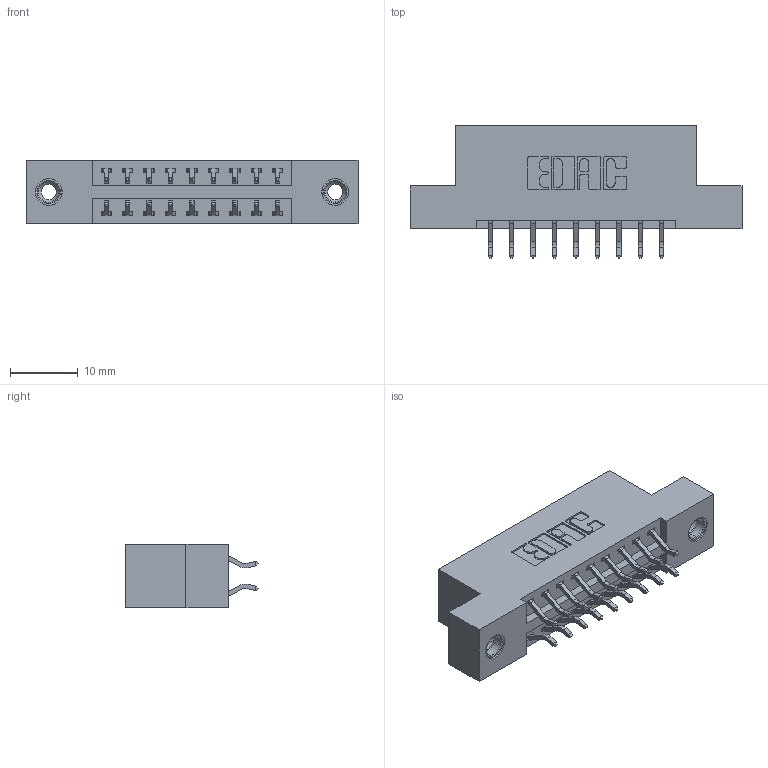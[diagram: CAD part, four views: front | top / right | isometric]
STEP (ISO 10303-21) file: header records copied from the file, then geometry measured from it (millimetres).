
FILE_DESCRIPTION (( 'STEP AP203' ), '1' );
FILE_NAME ('346-018-556-208.STEP', '2022-05-18T17:55:32', ( '' ), ( '' ), 'SwSTEP 2.0', 'SolidWorks 2020', '' );
FILE_SCHEMA (( 'CONFIG_CONTROL_DESIGN' ));
Length unit declared in the file: inch
Products named in the file (4): 346 Part_Flush Mounting Lugs - 0.156 Dia-TI; 345-292-001_556 Tail; 346-018-556-208; 345-250-001_345-250-003-102
Assembly tree (21 placements, depth 2):
  346-018-556-208
    346 Part_Flush Mounting Lugs - 0.156 Dia-TI
    345-292-001_556 Tail  x18
    345-250-001_345-250-003-102  x2
Bounding box: 49.15 x 19.57 x 9.4 mm (x, y, z)
Volume: 4529.1 mm3; surface area: 5710.2 mm2
Topology: 21 solids, 21 shells, 1226 faces, 3579 edges, 2354 vertices
Faces by surface type: plane 810, cylinder 400, cone 12, torus 4
Entity records: 11722 total; most frequent: CARTESIAN_POINT 1975, ORIENTED_EDGE 1890, DIRECTION 1807, EDGE_CURVE 945, LINE 749, VECTOR 749, VERTEX_POINT 624, AXIS2_PLACEMENT_3D 529
